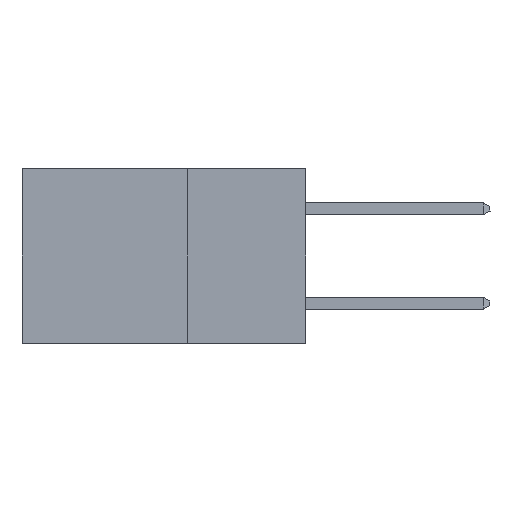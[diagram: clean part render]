
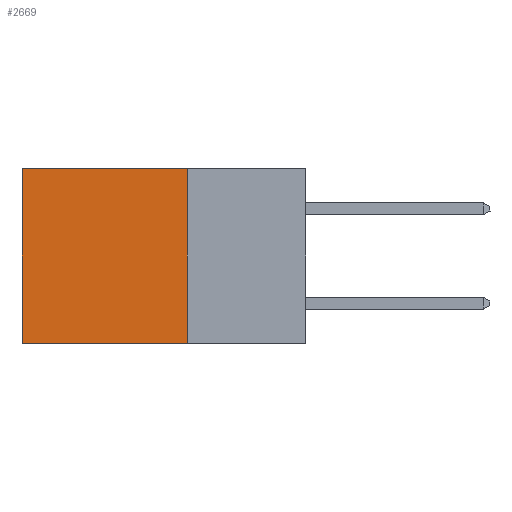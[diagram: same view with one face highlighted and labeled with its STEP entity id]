
A CAD part, left-side view. The second image highlights one B-rep face of the part: STEP entity #2669.
In plain terms, the highlighted planar face has unit normal (-1, 0, 0).
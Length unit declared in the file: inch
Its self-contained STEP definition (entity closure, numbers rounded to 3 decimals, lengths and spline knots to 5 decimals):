
#416 = CARTESIAN_POINT ( 'NONE',  ( 0.298, 0.25, 0. ) ) ;
#2044 = VECTOR ( 'NONE', #15399, 39.37008 ) ;
#2383 = EDGE_CURVE ( 'NONE', #2691, #8702, #19014, .T. ) ;
#2391 = DIRECTION ( 'NONE',  ( 0., 0., -1. ) ) ;
#2658 = LINE ( 'NONE', #23188, #8043 ) ;
#2669 = ADVANCED_FACE ( 'NONE', ( #16321 ), #12219, .F. ) ;
#2691 = VERTEX_POINT ( 'NONE', #9690 ) ;
#5001 = EDGE_CURVE ( 'NONE', #25641, #8702, #2658, .T. ) ;
#5079 = CARTESIAN_POINT ( 'NONE',  ( 0.298, 0.25, -0.37 ) ) ;
#6601 = ORIENTED_EDGE ( 'NONE', *, *, #19730, .F. ) ;
#8043 = VECTOR ( 'NONE', #10862, 39.37008 ) ;
#8647 = CARTESIAN_POINT ( 'NONE',  ( 0.298, 0.25, 0. ) ) ;
#8702 = VERTEX_POINT ( 'NONE', #15896 ) ;
#9690 = CARTESIAN_POINT ( 'NONE',  ( 0.298, 0.6, 0. ) ) ;
#10275 = EDGE_LOOP ( 'NONE', ( #18483, #23068, #6601, #19691 ) ) ;
#10310 = DIRECTION ( 'NONE',  ( 0., 0., -1. ) ) ;
#10339 = DIRECTION ( 'NONE',  ( 0., 1., 0. ) ) ;
#10446 = CARTESIAN_POINT ( 'NONE',  ( 0.298, 0.25, 0. ) ) ;
#10862 = DIRECTION ( 'NONE',  ( 0., 1., 0. ) ) ;
#12219 = PLANE ( 'NONE',  #28181 ) ;
#12238 = LINE ( 'NONE', #10446, #28462 ) ;
#12524 = VERTEX_POINT ( 'NONE', #8647 ) ;
#14718 = CARTESIAN_POINT ( 'NONE',  ( 0.298, 0.25, 0. ) ) ;
#14824 = VECTOR ( 'NONE', #10310, 39.37008 ) ;
#15399 = DIRECTION ( 'NONE',  ( 0., 0., -1. ) ) ;
#15896 = CARTESIAN_POINT ( 'NONE',  ( 0.298, 0.6, -0.37 ) ) ;
#16321 = FACE_OUTER_BOUND ( 'NONE', #10275, .T. ) ;
#18483 = ORIENTED_EDGE ( 'NONE', *, *, #2383, .T. ) ;
#19014 = LINE ( 'NONE', #30059, #2044 ) ;
#19668 = DIRECTION ( 'NONE',  ( 1., 0., 0. ) ) ;
#19691 = ORIENTED_EDGE ( 'NONE', *, *, #26547, .T. ) ;
#19730 = EDGE_CURVE ( 'NONE', #12524, #25641, #24455, .T. ) ;
#23068 = ORIENTED_EDGE ( 'NONE', *, *, #5001, .F. ) ;
#23188 = CARTESIAN_POINT ( 'NONE',  ( 0.298, 0.25, -0.37 ) ) ;
#24455 = LINE ( 'NONE', #416, #14824 ) ;
#25641 = VERTEX_POINT ( 'NONE', #5079 ) ;
#26547 = EDGE_CURVE ( 'NONE', #12524, #2691, #12238, .T. ) ;
#28181 = AXIS2_PLACEMENT_3D ( 'NONE', #14718, #19668, #2391 ) ;
#28462 = VECTOR ( 'NONE', #10339, 39.37008 ) ;
#30059 = CARTESIAN_POINT ( 'NONE',  ( 0.298, 0.6, 0. ) ) ;
